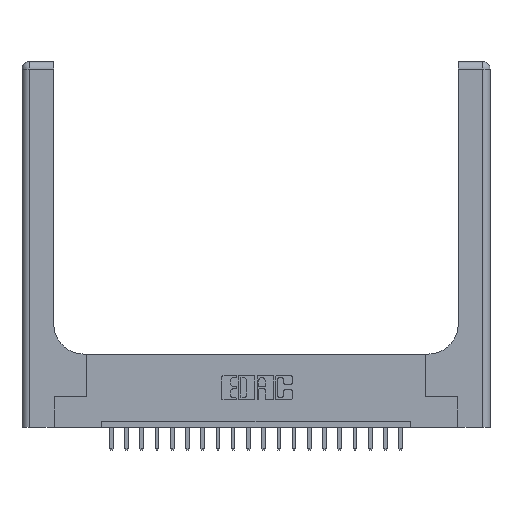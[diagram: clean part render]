
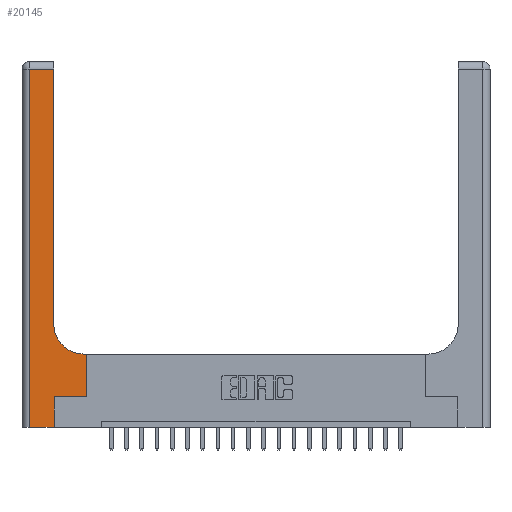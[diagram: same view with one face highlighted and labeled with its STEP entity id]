
A CAD part, top view. The second image highlights one B-rep face of the part: STEP entity #20145.
In plain terms, the highlighted planar face has unit normal (0, 0, 1).
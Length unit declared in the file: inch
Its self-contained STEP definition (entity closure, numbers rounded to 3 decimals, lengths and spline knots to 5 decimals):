
#16 = CARTESIAN_POINT ( 'NONE',  ( 0.528, 0.25, 0.37 ) ) ;
#473 = LINE ( 'NONE', #10177, #7844 ) ;
#503 = ORIENTED_EDGE ( 'NONE', *, *, #19196, .T. ) ;
#1164 = VERTEX_POINT ( 'NONE', #2313 ) ;
#1191 = CARTESIAN_POINT ( 'NONE',  ( 0., 2.94, 0.37 ) ) ;
#1228 = CARTESIAN_POINT ( 'NONE',  ( 0.528, 0.25, 0.37 ) ) ;
#1929 = VERTEX_POINT ( 'NONE', #13756 ) ;
#2066 = CARTESIAN_POINT ( 'NONE',  ( 0.51, 0.6, 0.37 ) ) ;
#2313 = CARTESIAN_POINT ( 'NONE',  ( 0.265, 0.25, 0.37 ) ) ;
#2616 = DIRECTION ( 'NONE',  ( -1., 0., 0. ) ) ;
#2975 = VERTEX_POINT ( 'NONE', #3737 ) ;
#3266 = DIRECTION ( 'NONE',  ( 0., 0., -1. ) ) ;
#3737 = CARTESIAN_POINT ( 'NONE',  ( 0.06, 2.94, 0.37 ) ) ;
#3776 = EDGE_CURVE ( 'NONE', #20689, #7151, #16178, .T. ) ;
#3988 = ORIENTED_EDGE ( 'NONE', *, *, #5794, .T. ) ;
#4152 = CARTESIAN_POINT ( 'NONE',  ( 0.265, 0., 0.37 ) ) ;
#4938 = ORIENTED_EDGE ( 'NONE', *, *, #3776, .T. ) ;
#4990 = DIRECTION ( 'NONE',  ( -1., 0., 0. ) ) ;
#5794 = EDGE_CURVE ( 'NONE', #14482, #6431, #19769, .T. ) ;
#6172 = ORIENTED_EDGE ( 'NONE', *, *, #11525, .T. ) ;
#6185 = DIRECTION ( 'NONE',  ( 0., 1., 0. ) ) ;
#6431 = VERTEX_POINT ( 'NONE', #4152 ) ;
#6588 = CARTESIAN_POINT ( 'NONE',  ( 0., 3., 0.37 ) ) ;
#6722 = EDGE_CURVE ( 'NONE', #1164, #15937, #11827, .T. ) ;
#7014 = CARTESIAN_POINT ( 'NONE',  ( 0.265, 0.25, 0.37 ) ) ;
#7151 = VERTEX_POINT ( 'NONE', #11692 ) ;
#7844 = VECTOR ( 'NONE', #15169, 39.37008 ) ;
#7888 = EDGE_CURVE ( 'NONE', #15937, #20517, #17834, .T. ) ;
#8613 = EDGE_CURVE ( 'NONE', #7151, #1929, #20457, .T. ) ;
#9204 = ORIENTED_EDGE ( 'NONE', *, *, #8613, .T. ) ;
#9363 = AXIS2_PLACEMENT_3D ( 'NONE', #16503, #3266, #14564 ) ;
#9410 = CARTESIAN_POINT ( 'NONE',  ( 0.26, 3., 0.37 ) ) ;
#9913 = EDGE_CURVE ( 'NONE', #1929, #2975, #11011, .T. ) ;
#10000 = PLANE ( 'NONE',  #17439 ) ;
#10067 = ORIENTED_EDGE ( 'NONE', *, *, #7888, .T. ) ;
#10177 = CARTESIAN_POINT ( 'NONE',  ( 0.265, 0., 0.37 ) ) ;
#10441 = VECTOR ( 'NONE', #13618, 39.37008 ) ;
#10653 = CARTESIAN_POINT ( 'NONE',  ( 0.06, 3., 0.37 ) ) ;
#10706 = EDGE_CURVE ( 'NONE', #2975, #14482, #13425, .T. ) ;
#11011 = LINE ( 'NONE', #1191, #16319 ) ;
#11525 = EDGE_CURVE ( 'NONE', #6431, #1164, #473, .T. ) ;
#11692 = CARTESIAN_POINT ( 'NONE',  ( 0.26, 0.85, 0.37 ) ) ;
#11827 = LINE ( 'NONE', #7014, #10441 ) ;
#13425 = LINE ( 'NONE', #10653, #14282 ) ;
#13618 = DIRECTION ( 'NONE',  ( 1., 0., 0. ) ) ;
#13662 = VECTOR ( 'NONE', #2616, 39.37008 ) ;
#13756 = CARTESIAN_POINT ( 'NONE',  ( 0.26, 2.94, 0.37 ) ) ;
#14031 = CARTESIAN_POINT ( 'NONE',  ( 0.528, 0.6, 0.37 ) ) ;
#14282 = VECTOR ( 'NONE', #18561, 39.37008 ) ;
#14465 = CARTESIAN_POINT ( 'NONE',  ( 0.06, 0., 0.37 ) ) ;
#14482 = VERTEX_POINT ( 'NONE', #14465 ) ;
#14564 = DIRECTION ( 'NONE',  ( 1., 0., 0. ) ) ;
#15169 = DIRECTION ( 'NONE',  ( 0., 1., 0. ) ) ;
#15270 = EDGE_LOOP ( 'NONE', ( #9204, #16580, #17285, #3988, #6172, #18316, #10067, #503, #4938 ) ) ;
#15914 = DIRECTION ( 'NONE',  ( 0., 1., 0. ) ) ;
#15937 = VERTEX_POINT ( 'NONE', #1228 ) ;
#16063 = DIRECTION ( 'NONE',  ( 0., 0., -1. ) ) ;
#16178 = CIRCLE ( 'NONE', #9363, 0.25 ) ;
#16319 = VECTOR ( 'NONE', #20641, 39.37008 ) ;
#16503 = CARTESIAN_POINT ( 'NONE',  ( 0.51, 0.85, 0.37 ) ) ;
#16580 = ORIENTED_EDGE ( 'NONE', *, *, #9913, .T. ) ;
#16602 = VECTOR ( 'NONE', #18151, 39.37008 ) ;
#16749 = CARTESIAN_POINT ( 'NONE',  ( 0., 0., 0.37 ) ) ;
#17247 = LINE ( 'NONE', #17440, #13662 ) ;
#17285 = ORIENTED_EDGE ( 'NONE', *, *, #10706, .T. ) ;
#17439 = AXIS2_PLACEMENT_3D ( 'NONE', #6588, #16063, #4990 ) ;
#17440 = CARTESIAN_POINT ( 'NONE',  ( 0.26, 0.6, 0.37 ) ) ;
#17834 = LINE ( 'NONE', #16, #19016 ) ;
#18002 = VECTOR ( 'NONE', #15914, 39.37008 ) ;
#18151 = DIRECTION ( 'NONE',  ( 1., 0., 0. ) ) ;
#18316 = ORIENTED_EDGE ( 'NONE', *, *, #6722, .T. ) ;
#18561 = DIRECTION ( 'NONE',  ( 0., -1., 0. ) ) ;
#19016 = VECTOR ( 'NONE', #6185, 39.37008 ) ;
#19196 = EDGE_CURVE ( 'NONE', #20517, #20689, #17247, .T. ) ;
#19736 = FACE_OUTER_BOUND ( 'NONE', #15270, .T. ) ;
#19769 = LINE ( 'NONE', #16749, #16602 ) ;
#20145 = ADVANCED_FACE ( 'NONE', ( #19736 ), #10000, .F. ) ;
#20457 = LINE ( 'NONE', #9410, #18002 ) ;
#20517 = VERTEX_POINT ( 'NONE', #14031 ) ;
#20641 = DIRECTION ( 'NONE',  ( -1., 0., 0. ) ) ;
#20689 = VERTEX_POINT ( 'NONE', #2066 ) ;
